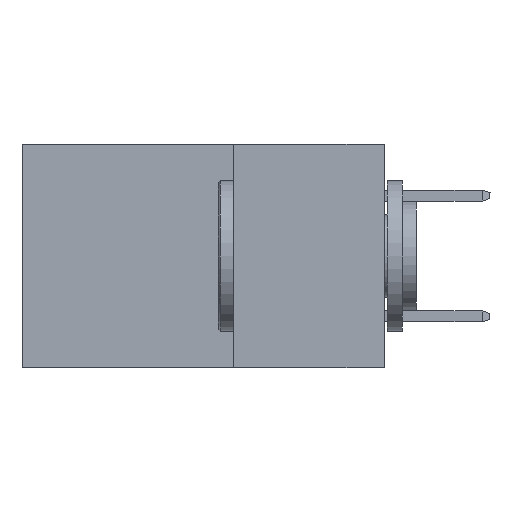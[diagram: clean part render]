
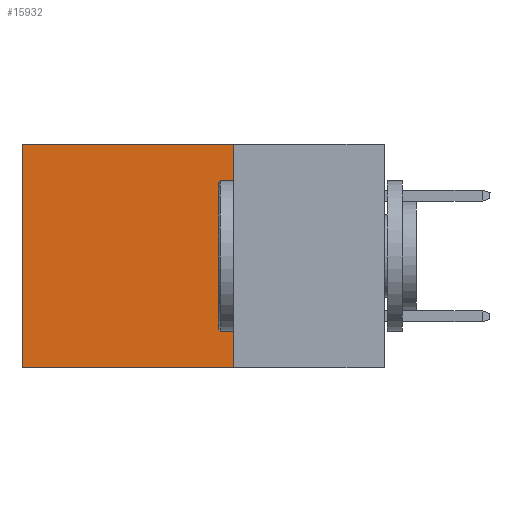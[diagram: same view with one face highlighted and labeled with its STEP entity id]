
A CAD part, left-side view. The second image highlights one B-rep face of the part: STEP entity #15932.
In plain terms, the highlighted planar face has unit normal (-1, 0, 0).
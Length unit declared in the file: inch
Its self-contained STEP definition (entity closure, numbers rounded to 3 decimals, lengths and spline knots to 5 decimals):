
#1660 = CARTESIAN_POINT ( 'NONE',  ( 0.2615, 0.6, 0. ) ) ;
#1769 = CARTESIAN_POINT ( 'NONE',  ( 0.2615, 0.25, -0.37 ) ) ;
#3621 = ORIENTED_EDGE ( 'NONE', *, *, #13326, .T. ) ;
#3730 = CARTESIAN_POINT ( 'NONE',  ( 0.2615, 0.6, -0.37 ) ) ;
#3933 = DIRECTION ( 'NONE',  ( 0., 1., 0. ) ) ;
#4275 = EDGE_CURVE ( 'NONE', #4296, #9400, #16577, .T. ) ;
#4296 = VERTEX_POINT ( 'NONE', #8181 ) ;
#5339 = VECTOR ( 'NONE', #8717, 39.37008 ) ;
#5559 = ORIENTED_EDGE ( 'NONE', *, *, #7668, .F. ) ;
#5810 = DIRECTION ( 'NONE',  ( 1., 0., 0. ) ) ;
#7668 = EDGE_CURVE ( 'NONE', #9400, #20613, #22179, .T. ) ;
#8036 = CARTESIAN_POINT ( 'NONE',  ( 0.2615, 0.6, -0.37 ) ) ;
#8181 = CARTESIAN_POINT ( 'NONE',  ( 0.2615, 0.25, 0. ) ) ;
#8315 = CARTESIAN_POINT ( 'NONE',  ( 0.2615, 0.25, -0.37 ) ) ;
#8717 = DIRECTION ( 'NONE',  ( 0., 0., -1. ) ) ;
#9400 = VERTEX_POINT ( 'NONE', #9849 ) ;
#9647 = CARTESIAN_POINT ( 'NONE',  ( 0.2615, 0.25, 0. ) ) ;
#9849 = CARTESIAN_POINT ( 'NONE',  ( 0.2615, 0.25, -0.37 ) ) ;
#10193 = VECTOR ( 'NONE', #22107, 39.37008 ) ;
#10304 = AXIS2_PLACEMENT_3D ( 'NONE', #18404, #5810, #20464 ) ;
#11135 = VECTOR ( 'NONE', #3933, 39.37008 ) ;
#12090 = PLANE ( 'NONE',  #10304 ) ;
#12745 = ORIENTED_EDGE ( 'NONE', *, *, #4275, .F. ) ;
#13326 = EDGE_CURVE ( 'NONE', #17390, #20613, #20892, .T. ) ;
#13882 = FACE_OUTER_BOUND ( 'NONE', #17578, .T. ) ;
#15932 = ADVANCED_FACE ( 'NONE', ( #13882 ), #12090, .F. ) ;
#16577 = LINE ( 'NONE', #8315, #5339 ) ;
#17231 = EDGE_CURVE ( 'NONE', #4296, #17390, #21260, .T. ) ;
#17390 = VERTEX_POINT ( 'NONE', #1660 ) ;
#17578 = EDGE_LOOP ( 'NONE', ( #3621, #5559, #12745, #17673 ) ) ;
#17673 = ORIENTED_EDGE ( 'NONE', *, *, #17231, .T. ) ;
#18404 = CARTESIAN_POINT ( 'NONE',  ( 0.2615, 0.25, -0.37 ) ) ;
#20464 = DIRECTION ( 'NONE',  ( 0., 0., -1. ) ) ;
#20613 = VERTEX_POINT ( 'NONE', #8036 ) ;
#20892 = LINE ( 'NONE', #3730, #22183 ) ;
#21260 = LINE ( 'NONE', #9647, #10193 ) ;
#22107 = DIRECTION ( 'NONE',  ( 0., 1., 0. ) ) ;
#22179 = LINE ( 'NONE', #1769, #11135 ) ;
#22183 = VECTOR ( 'NONE', #24750, 39.37008 ) ;
#24750 = DIRECTION ( 'NONE',  ( 0., 0., -1. ) ) ;
